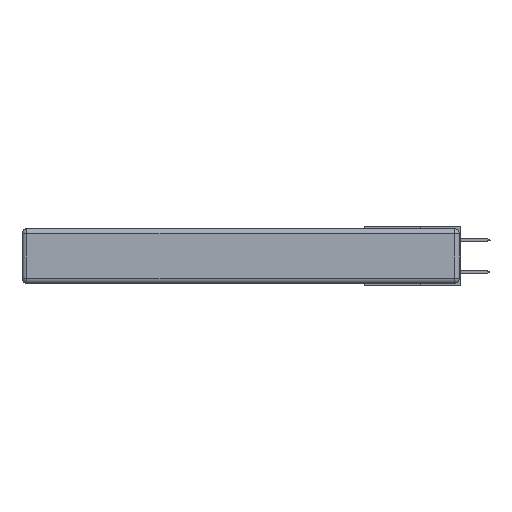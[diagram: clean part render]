
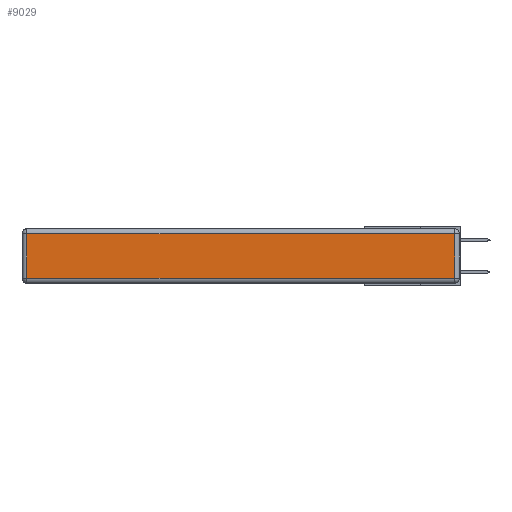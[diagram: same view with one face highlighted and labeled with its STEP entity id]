
A CAD part, left-side view. The second image highlights one B-rep face of the part: STEP entity #9029.
In plain terms, the highlighted planar face has unit normal (-1, 0, 0).
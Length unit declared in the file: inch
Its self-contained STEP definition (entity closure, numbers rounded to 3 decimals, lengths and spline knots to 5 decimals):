
#442 = VERTEX_POINT ( 'NONE', #2812 ) ;
#972 = EDGE_CURVE ( 'NONE', #15967, #8564, #1484, .T. ) ;
#1484 = LINE ( 'NONE', #8093, #22429 ) ;
#1733 = VECTOR ( 'NONE', #22778, 39.37008 ) ;
#1740 = VERTEX_POINT ( 'NONE', #8899 ) ;
#1843 = DIRECTION ( 'NONE',  ( 0., -1., 0. ) ) ;
#2265 = DIRECTION ( 'NONE',  ( 0., 1., 0. ) ) ;
#2614 = EDGE_CURVE ( 'NONE', #8564, #442, #12016, .T. ) ;
#2812 = CARTESIAN_POINT ( 'NONE',  ( 0., 2.72, -0.313 ) ) ;
#5473 = DIRECTION ( 'NONE',  ( -1., 0., 0. ) ) ;
#7523 = DIRECTION ( 'NONE',  ( 0., 0., 1. ) ) ;
#8032 = AXIS2_PLACEMENT_3D ( 'NONE', #15290, #5473, #18904 ) ;
#8093 = CARTESIAN_POINT ( 'NONE',  ( 0., 2.75, -0.03 ) ) ;
#8564 = VERTEX_POINT ( 'NONE', #9120 ) ;
#8899 = CARTESIAN_POINT ( 'NONE',  ( 0., 0.03, -0.313 ) ) ;
#9029 = ADVANCED_FACE ( 'NONE', ( #13819 ), #25047, .T. ) ;
#9120 = CARTESIAN_POINT ( 'NONE',  ( 0., 2.72, -0.03 ) ) ;
#9535 = CARTESIAN_POINT ( 'NONE',  ( 0., 0., -0.313 ) ) ;
#9680 = VECTOR ( 'NONE', #1843, 39.37008 ) ;
#10092 = ORIENTED_EDGE ( 'NONE', *, *, #972, .T. ) ;
#10512 = EDGE_CURVE ( 'NONE', #442, #1740, #24302, .T. ) ;
#10980 = CARTESIAN_POINT ( 'NONE',  ( 0., 0.03, -0.03 ) ) ;
#12016 = LINE ( 'NONE', #22942, #1733 ) ;
#12396 = VECTOR ( 'NONE', #7523, 39.37008 ) ;
#13200 = ORIENTED_EDGE ( 'NONE', *, *, #2614, .T. ) ;
#13819 = FACE_OUTER_BOUND ( 'NONE', #16923, .T. ) ;
#15290 = CARTESIAN_POINT ( 'NONE',  ( 0., 0., -0.343 ) ) ;
#15321 = ORIENTED_EDGE ( 'NONE', *, *, #20217, .T. ) ;
#15474 = ORIENTED_EDGE ( 'NONE', *, *, #10512, .T. ) ;
#15967 = VERTEX_POINT ( 'NONE', #10980 ) ;
#16923 = EDGE_LOOP ( 'NONE', ( #15474, #15321, #10092, #13200 ) ) ;
#18904 = DIRECTION ( 'NONE',  ( 0., 0., 1. ) ) ;
#20217 = EDGE_CURVE ( 'NONE', #1740, #15967, #22744, .T. ) ;
#21099 = CARTESIAN_POINT ( 'NONE',  ( 0., 0.03, -0.343 ) ) ;
#22429 = VECTOR ( 'NONE', #2265, 39.37008 ) ;
#22744 = LINE ( 'NONE', #21099, #12396 ) ;
#22778 = DIRECTION ( 'NONE',  ( 0., 0., -1. ) ) ;
#22942 = CARTESIAN_POINT ( 'NONE',  ( 0., 2.72, -0.343 ) ) ;
#24302 = LINE ( 'NONE', #9535, #9680 ) ;
#25047 = PLANE ( 'NONE',  #8032 ) ;
